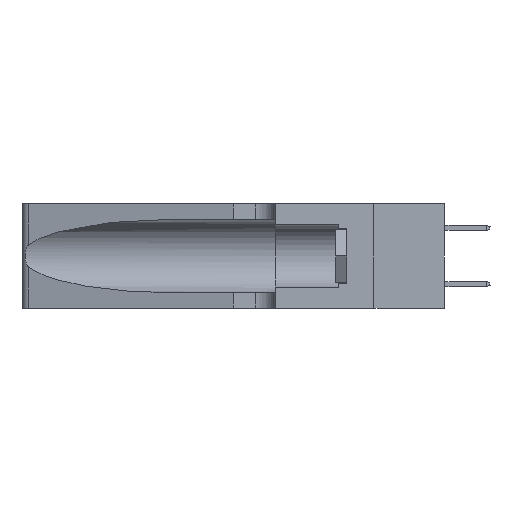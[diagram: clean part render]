
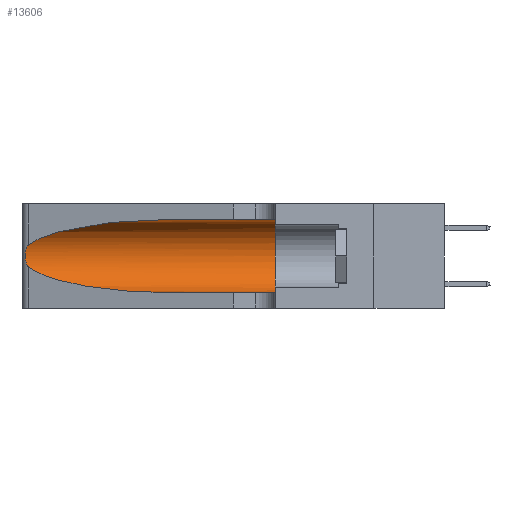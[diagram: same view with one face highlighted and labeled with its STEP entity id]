
A CAD part, left-side view. The second image highlights one B-rep face of the part: STEP entity #13606.
In plain terms, the highlighted cylindrical face has radius 3.308 mm (diameter 6.617 mm), a partial arc.
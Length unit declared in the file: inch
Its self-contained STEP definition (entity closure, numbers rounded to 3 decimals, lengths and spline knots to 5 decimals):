
#27 = FACE_OUTER_BOUND ( 'NONE', #35888, .T. ) ;
#63 = ORIENTED_EDGE ( 'NONE', *, *, #19292, .T. ) ;
#136 = AXIS2_PLACEMENT_3D ( 'NONE', #21982, #15779, #3772 ) ;
#992 = VERTEX_POINT ( 'NONE', #38423 ) ;
#1155 = CARTESIAN_POINT ( 'NONE',  ( 0.25487, 1.22718, 0.14631 ) ) ;
#1485 = LINE ( 'NONE', #27798, #32184 ) ;
#2136 = LINE ( 'NONE', #16418, #9274 ) ;
#2908 = CARTESIAN_POINT ( 'NONE',  ( 0.1305, 0.35, 0.05475 ) ) ;
#3772 = DIRECTION ( 'NONE',  ( 0., 0., 1. ) ) ;
#3856 =( BOUNDED_CURVE ( )  B_SPLINE_CURVE ( 3, ( #38940, #11369, #8540, #32821 ),
 .UNSPECIFIED., .F., .T. ) 
 B_SPLINE_CURVE_WITH_KNOTS ( ( 4, 4 ),
 ( 1.5708, 2.84003 ),
 .UNSPECIFIED. ) 
 CURVE ( )  GEOMETRIC_REPRESENTATION_ITEM ( )  RATIONAL_B_SPLINE_CURVE ( ( 1., 0.87, 0.87, 1. ) ) 
 REPRESENTATION_ITEM ( '' )  );
#5559 = VERTEX_POINT ( 'NONE', #2908 ) ;
#5723 = VERTEX_POINT ( 'NONE', #21748 ) ;
#7652 = CIRCLE ( 'NONE', #136, 0.13025 ) ;
#8540 = CARTESIAN_POINT ( 'NONE',  ( 0.2373, 1.15595, 0.28018 ) ) ;
#8588 = CARTESIAN_POINT ( 'NONE',  ( 0.1305, 1.61858, 0.185 ) ) ;
#8752 = CARTESIAN_POINT ( 'NONE',  ( 0.1305, 0.72297, 0.05475 ) ) ;
#9274 = VECTOR ( 'NONE', #21425, 39.37008 ) ;
#10175 = EDGE_CURVE ( 'NONE', #5723, #24948, #1485, .T. ) ;
#11304 = ORIENTED_EDGE ( 'NONE', *, *, #10175, .F. ) ;
#11369 = CARTESIAN_POINT ( 'NONE',  ( 0.18966, 0.96281, 0.31525 ) ) ;
#13606 = ADVANCED_FACE ( 'NONE', ( #27 ), #31632, .F. ) ;
#13898 = CARTESIAN_POINT ( 'NONE',  ( 0.25487, 1.22718, 0.22369 ) ) ;
#15779 = DIRECTION ( 'NONE',  ( 0., 1., 0. ) ) ;
#16110 = DIRECTION ( 'NONE',  ( 0., -1., 0. ) ) ;
#16418 = CARTESIAN_POINT ( 'NONE',  ( 0.1305, 1.61858, 0.05475 ) ) ;
#16990 = CARTESIAN_POINT ( 'NONE',  ( 0.26018, 1.23835, 0.19895 ) ) ;
#19292 = EDGE_CURVE ( 'NONE', #20496, #31754, #24786, .T. ) ;
#19628 = CARTESIAN_POINT ( 'NONE',  ( 0.25555, 1.22993, 0.14849 ) ) ;
#19688 = EDGE_CURVE ( 'NONE', #992, #5559, #2136, .T. ) ;
#19927 = CARTESIAN_POINT ( 'NONE',  ( 0.25487, 1.22718, 0.22369 ) ) ;
#20090 = CARTESIAN_POINT ( 'NONE',  ( 0.26075, 1.23896, 0.19203 ) ) ;
#20496 = VERTEX_POINT ( 'NONE', #19927 ) ;
#20505 = CARTESIAN_POINT ( 'NONE',  ( 0.25555, 1.22994, 0.2215 ) ) ;
#20584 = CARTESIAN_POINT ( 'NONE',  ( 0.1305, 0.35, 0.31525 ) ) ;
#20922 = DIRECTION ( 'NONE',  ( 0., 0., -1. ) ) ;
#21052 = DIRECTION ( 'NONE',  ( 0., -1., 0. ) ) ;
#21425 = DIRECTION ( 'NONE',  ( 0., -1., 0. ) ) ;
#21536 = EDGE_CURVE ( 'NONE', #24948, #5559, #7652, .T. ) ;
#21748 = CARTESIAN_POINT ( 'NONE',  ( 0.1305, 0.72297, 0.31525 ) ) ;
#21982 = CARTESIAN_POINT ( 'NONE',  ( 0.1305, 0.35, 0.185 ) ) ;
#23070 = ORIENTED_EDGE ( 'NONE', *, *, #24114, .T. ) ;
#23175 = CARTESIAN_POINT ( 'NONE',  ( 0.25856, 1.23593, 0.16098 ) ) ;
#24114 = EDGE_CURVE ( 'NONE', #31754, #992, #30687, .T. ) ;
#24786 = B_SPLINE_CURVE_WITH_KNOTS ( 'NONE', 3,
 ( #13898, #20505, #35428, #26171, #38554, #16990, #20090, #26311, #34834, #23175, #38504, #32135, #19628, #1155 ),
 .UNSPECIFIED., .F., .F.,
 ( 4, 2, 2, 2, 2, 2, 4 ),
 ( 0., 0.00027, 0.00053, 0.00107, 0.0016, 0.00187, 0.00214 ),
 .UNSPECIFIED. ) ;
#24948 = VERTEX_POINT ( 'NONE', #20584 ) ;
#25204 = ORIENTED_EDGE ( 'NONE', *, *, #21536, .F. ) ;
#26171 = CARTESIAN_POINT ( 'NONE',  ( 0.25787, 1.23484, 0.2124 ) ) ;
#26311 = CARTESIAN_POINT ( 'NONE',  ( 0.26075, 1.23896, 0.178 ) ) ;
#27798 = CARTESIAN_POINT ( 'NONE',  ( 0.1305, 1.61858, 0.31525 ) ) ;
#28519 = ORIENTED_EDGE ( 'NONE', *, *, #19688, .T. ) ;
#29511 = AXIS2_PLACEMENT_3D ( 'NONE', #8588, #21052, #20922 ) ;
#29836 = CARTESIAN_POINT ( 'NONE',  ( 0.25487, 1.22718, 0.14631 ) ) ;
#30687 =( BOUNDED_CURVE ( )  B_SPLINE_CURVE ( 3, ( #29836, #39416, #30756, #8752 ),
 .UNSPECIFIED., .F., .T. ) 
 B_SPLINE_CURVE_WITH_KNOTS ( ( 4, 4 ),
 ( 3.44316, 4.71239 ),
 .UNSPECIFIED. ) 
 CURVE ( )  GEOMETRIC_REPRESENTATION_ITEM ( )  RATIONAL_B_SPLINE_CURVE ( ( 1., 0.87, 0.87, 1. ) ) 
 REPRESENTATION_ITEM ( '' )  );
#30756 = CARTESIAN_POINT ( 'NONE',  ( 0.18966, 0.96281, 0.05475 ) ) ;
#31632 = CYLINDRICAL_SURFACE ( 'NONE', #29511, 0.13025 ) ;
#31754 = VERTEX_POINT ( 'NONE', #39491 ) ;
#32135 = CARTESIAN_POINT ( 'NONE',  ( 0.25639, 1.23186, 0.15144 ) ) ;
#32184 = VECTOR ( 'NONE', #16110, 39.37008 ) ;
#32821 = CARTESIAN_POINT ( 'NONE',  ( 0.25487, 1.22718, 0.22369 ) ) ;
#32914 = EDGE_CURVE ( 'NONE', #5723, #20496, #3856, .T. ) ;
#34834 = CARTESIAN_POINT ( 'NONE',  ( 0.26017, 1.23833, 0.17102 ) ) ;
#35377 = ORIENTED_EDGE ( 'NONE', *, *, #32914, .T. ) ;
#35428 = CARTESIAN_POINT ( 'NONE',  ( 0.25639, 1.23184, 0.21858 ) ) ;
#35888 = EDGE_LOOP ( 'NONE', ( #35377, #63, #23070, #28519, #25204, #11304 ) ) ;
#38423 = CARTESIAN_POINT ( 'NONE',  ( 0.1305, 0.72297, 0.05475 ) ) ;
#38504 = CARTESIAN_POINT ( 'NONE',  ( 0.25789, 1.23486, 0.15765 ) ) ;
#38554 = CARTESIAN_POINT ( 'NONE',  ( 0.25854, 1.2359, 0.20912 ) ) ;
#38940 = CARTESIAN_POINT ( 'NONE',  ( 0.1305, 0.72297, 0.31525 ) ) ;
#39416 = CARTESIAN_POINT ( 'NONE',  ( 0.2373, 1.15595, 0.08982 ) ) ;
#39491 = CARTESIAN_POINT ( 'NONE',  ( 0.25487, 1.22718, 0.14631 ) ) ;
